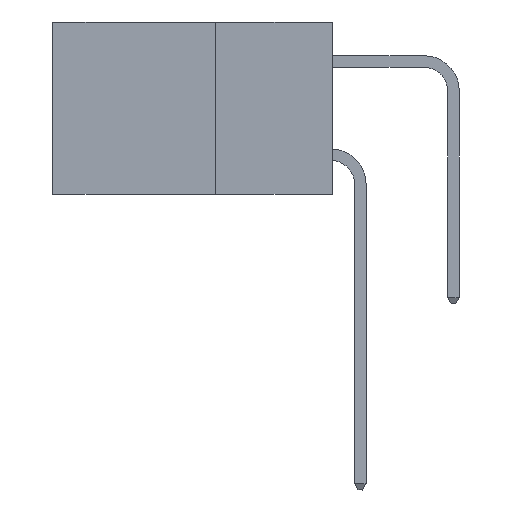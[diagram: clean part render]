
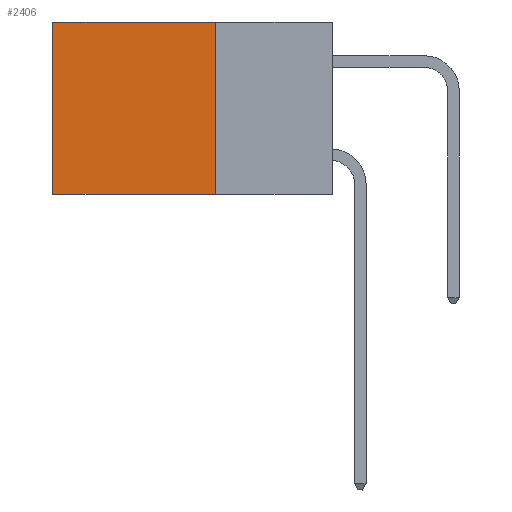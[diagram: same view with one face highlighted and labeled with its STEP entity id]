
A CAD part, left-side view. The second image highlights one B-rep face of the part: STEP entity #2406.
In plain terms, the highlighted planar face has unit normal (-1, 0, 0).
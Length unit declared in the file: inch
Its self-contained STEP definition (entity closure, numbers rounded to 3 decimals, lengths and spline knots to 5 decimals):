
#192 = VECTOR ( 'NONE', #31039, 39.37008 ) ;
#671 = DIRECTION ( 'NONE',  ( 1., 0., 0. ) ) ;
#1526 = CARTESIAN_POINT ( 'NONE',  ( 0.298, 0.25, 0. ) ) ;
#1954 = VERTEX_POINT ( 'NONE', #4481 ) ;
#2406 = ADVANCED_FACE ( 'NONE', ( #4709 ), #2491, .F. ) ;
#2479 = LINE ( 'NONE', #4474, #192 ) ;
#2491 = PLANE ( 'NONE',  #24437 ) ;
#3248 = CARTESIAN_POINT ( 'NONE',  ( 0.298, 0.25, 0. ) ) ;
#3658 = EDGE_CURVE ( 'NONE', #11402, #14354, #29426, .T. ) ;
#4474 = CARTESIAN_POINT ( 'NONE',  ( 0.298, 0.25, -0.37 ) ) ;
#4481 = CARTESIAN_POINT ( 'NONE',  ( 0.298, 0.25, -0.37 ) ) ;
#4709 = FACE_OUTER_BOUND ( 'NONE', #13201, .T. ) ;
#7833 = EDGE_CURVE ( 'NONE', #1954, #13866, #2479, .T. ) ;
#10237 = CARTESIAN_POINT ( 'NONE',  ( 0.298, 0.25, 0. ) ) ;
#10562 = ORIENTED_EDGE ( 'NONE', *, *, #3658, .T. ) ;
#10683 = DIRECTION ( 'NONE',  ( 0., 1., 0. ) ) ;
#11330 = CARTESIAN_POINT ( 'NONE',  ( 0.298, 0.6, 0. ) ) ;
#11402 = VERTEX_POINT ( 'NONE', #3248 ) ;
#12334 = VECTOR ( 'NONE', #30162, 39.37008 ) ;
#13201 = EDGE_LOOP ( 'NONE', ( #22474, #28208, #24036, #10562 ) ) ;
#13866 = VERTEX_POINT ( 'NONE', #16391 ) ;
#14354 = VERTEX_POINT ( 'NONE', #26283 ) ;
#14706 = EDGE_CURVE ( 'NONE', #14354, #13866, #26204, .T. ) ;
#15250 = LINE ( 'NONE', #29719, #30608 ) ;
#16391 = CARTESIAN_POINT ( 'NONE',  ( 0.298, 0.6, -0.37 ) ) ;
#16674 = VECTOR ( 'NONE', #10683, 39.37008 ) ;
#17606 = DIRECTION ( 'NONE',  ( 0., 0., -1. ) ) ;
#19830 = EDGE_CURVE ( 'NONE', #11402, #1954, #15250, .T. ) ;
#22179 = DIRECTION ( 'NONE',  ( 0., 0., -1. ) ) ;
#22474 = ORIENTED_EDGE ( 'NONE', *, *, #14706, .T. ) ;
#24036 = ORIENTED_EDGE ( 'NONE', *, *, #19830, .F. ) ;
#24437 = AXIS2_PLACEMENT_3D ( 'NONE', #10237, #671, #22179 ) ;
#26204 = LINE ( 'NONE', #11330, #12334 ) ;
#26283 = CARTESIAN_POINT ( 'NONE',  ( 0.298, 0.6, 0. ) ) ;
#28208 = ORIENTED_EDGE ( 'NONE', *, *, #7833, .F. ) ;
#29426 = LINE ( 'NONE', #1526, #16674 ) ;
#29719 = CARTESIAN_POINT ( 'NONE',  ( 0.298, 0.25, 0. ) ) ;
#30162 = DIRECTION ( 'NONE',  ( 0., 0., -1. ) ) ;
#30608 = VECTOR ( 'NONE', #17606, 39.37008 ) ;
#31039 = DIRECTION ( 'NONE',  ( 0., 1., 0. ) ) ;
